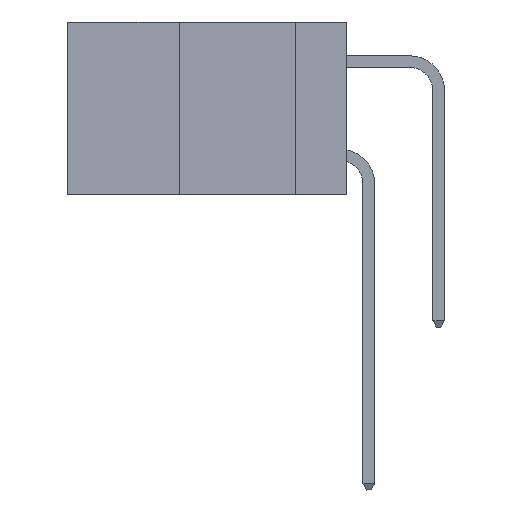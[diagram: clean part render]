
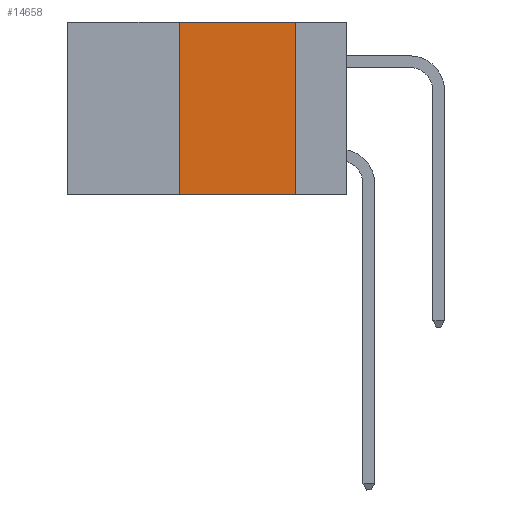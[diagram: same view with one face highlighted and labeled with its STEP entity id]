
A CAD part, left-side view. The second image highlights one B-rep face of the part: STEP entity #14658.
In plain terms, the highlighted planar face has unit normal (-1, 0, 0).
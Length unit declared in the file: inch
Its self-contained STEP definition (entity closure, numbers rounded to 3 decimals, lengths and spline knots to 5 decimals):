
#185 = EDGE_CURVE ( 'NONE', #20866, #217, #18952, .T. ) ;
#217 = VERTEX_POINT ( 'NONE', #9396 ) ;
#1453 = VERTEX_POINT ( 'NONE', #7879 ) ;
#1549 = CARTESIAN_POINT ( 'NONE',  ( 0., 0.36, -0.37 ) ) ;
#1609 = EDGE_CURVE ( 'NONE', #10400, #1453, #4488, .T. ) ;
#3722 = ORIENTED_EDGE ( 'NONE', *, *, #1609, .T. ) ;
#3996 = VECTOR ( 'NONE', #14615, 39.37008 ) ;
#4337 = EDGE_CURVE ( 'NONE', #217, #1453, #6266, .T. ) ;
#4488 = LINE ( 'NONE', #8263, #3996 ) ;
#4747 = DIRECTION ( 'NONE',  ( 0., 0., -1. ) ) ;
#6266 = LINE ( 'NONE', #15352, #10120 ) ;
#6473 = CARTESIAN_POINT ( 'NONE',  ( 0., 0.6, 0. ) ) ;
#7292 = DIRECTION ( 'NONE',  ( 0., 0., -1. ) ) ;
#7792 = EDGE_CURVE ( 'NONE', #10400, #20866, #14003, .T. ) ;
#7879 = CARTESIAN_POINT ( 'NONE',  ( 0., 0.11, -0.37 ) ) ;
#8061 = DIRECTION ( 'NONE',  ( 0., -1., 0. ) ) ;
#8263 = CARTESIAN_POINT ( 'NONE',  ( 0., 0.6, -0.37 ) ) ;
#9396 = CARTESIAN_POINT ( 'NONE',  ( 0., 0.11, 0. ) ) ;
#9444 = CARTESIAN_POINT ( 'NONE',  ( 0., 0.36, 0. ) ) ;
#9696 = VECTOR ( 'NONE', #16637, 39.37008 ) ;
#10120 = VECTOR ( 'NONE', #7292, 39.37008 ) ;
#10400 = VERTEX_POINT ( 'NONE', #1549 ) ;
#11228 = PLANE ( 'NONE',  #13497 ) ;
#12431 = ORIENTED_EDGE ( 'NONE', *, *, #185, .F. ) ;
#12918 = CARTESIAN_POINT ( 'NONE',  ( 0., 0.6, 0. ) ) ;
#13397 = EDGE_LOOP ( 'NONE', ( #18601, #12431, #14915, #3722 ) ) ;
#13497 = AXIS2_PLACEMENT_3D ( 'NONE', #12918, #14537, #4747 ) ;
#14003 = LINE ( 'NONE', #15064, #9696 ) ;
#14537 = DIRECTION ( 'NONE',  ( 1., 0., 0. ) ) ;
#14615 = DIRECTION ( 'NONE',  ( 0., -1., 0. ) ) ;
#14658 = ADVANCED_FACE ( 'NONE', ( #20737 ), #11228, .F. ) ;
#14771 = VECTOR ( 'NONE', #8061, 39.37008 ) ;
#14915 = ORIENTED_EDGE ( 'NONE', *, *, #7792, .F. ) ;
#15064 = CARTESIAN_POINT ( 'NONE',  ( 0., 0.36, 0. ) ) ;
#15352 = CARTESIAN_POINT ( 'NONE',  ( 0., 0.11, 0. ) ) ;
#16637 = DIRECTION ( 'NONE',  ( 0., 0., 1. ) ) ;
#18601 = ORIENTED_EDGE ( 'NONE', *, *, #4337, .F. ) ;
#18952 = LINE ( 'NONE', #6473, #14771 ) ;
#20737 = FACE_OUTER_BOUND ( 'NONE', #13397, .T. ) ;
#20866 = VERTEX_POINT ( 'NONE', #9444 ) ;
